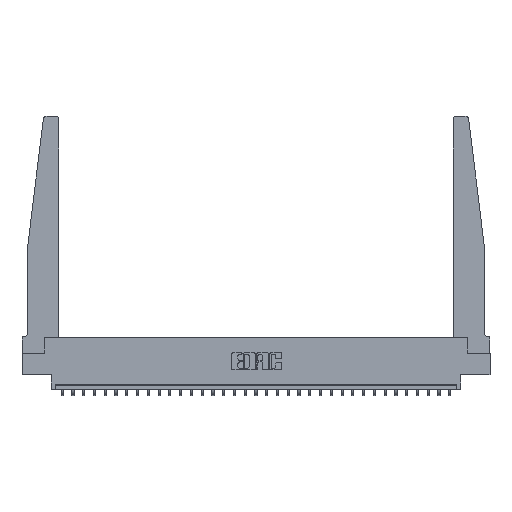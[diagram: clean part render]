
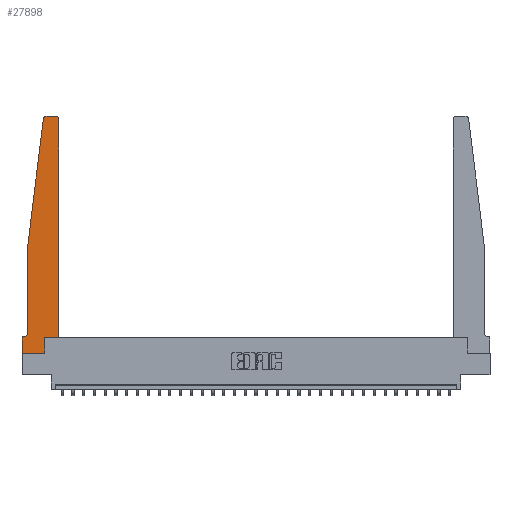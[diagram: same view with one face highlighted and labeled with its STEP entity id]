
A CAD part, top view. The second image highlights one B-rep face of the part: STEP entity #27898.
In plain terms, the highlighted planar face has unit normal (0, 0, 1).
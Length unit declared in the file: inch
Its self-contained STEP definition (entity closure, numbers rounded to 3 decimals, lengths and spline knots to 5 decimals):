
#23 = CARTESIAN_POINT ( 'NONE',  ( 0.425, 0.18, 0.37 ) ) ;
#372 = ORIENTED_EDGE ( 'NONE', *, *, #11865, .T. ) ;
#1064 = CARTESIAN_POINT ( 'NONE',  ( 0., 0., 0.37 ) ) ;
#1239 = CARTESIAN_POINT ( 'NONE',  ( 0.065, 0.1875, 0.37 ) ) ;
#1518 = VECTOR ( 'NONE', #21437, 39.37008 ) ;
#2028 = ORIENTED_EDGE ( 'NONE', *, *, #18009, .T. ) ;
#2218 = FACE_OUTER_BOUND ( 'NONE', #23320, .T. ) ;
#2490 = CARTESIAN_POINT ( 'NONE',  ( 0., 0., 0.37 ) ) ;
#2788 = CARTESIAN_POINT ( 'NONE',  ( 0.395, 2.72, 0.37 ) ) ;
#3418 = ORIENTED_EDGE ( 'NONE', *, *, #25724, .T. ) ;
#3942 = CIRCLE ( 'NONE', #22882, 0.03 ) ;
#4179 = CARTESIAN_POINT ( 'NONE',  ( 0.015, 0.2375, 0.37 ) ) ;
#5084 = DIRECTION ( 'NONE',  ( 1., 0., 0. ) ) ;
#5441 = CIRCLE ( 'NONE', #22124, 0.05 ) ;
#5722 = VERTEX_POINT ( 'NONE', #16955 ) ;
#6026 = VECTOR ( 'NONE', #18475, 39.37008 ) ;
#6123 = CARTESIAN_POINT ( 'NONE',  ( 0.425, 0.18, 0.37 ) ) ;
#6219 = CARTESIAN_POINT ( 'NONE',  ( 0.25, 2.75, 0.37 ) ) ;
#6423 = DIRECTION ( 'NONE',  ( -1., 0., 0. ) ) ;
#6855 = DIRECTION ( 'NONE',  ( 0., 0., 1. ) ) ;
#7719 = EDGE_CURVE ( 'NONE', #25180, #16531, #5441, .T. ) ;
#7782 = ORIENTED_EDGE ( 'NONE', *, *, #21812, .T. ) ;
#7826 = LINE ( 'NONE', #6219, #13737 ) ;
#7830 = VERTEX_POINT ( 'NONE', #23 ) ;
#8105 = EDGE_CURVE ( 'NONE', #7830, #5722, #19169, .T. ) ;
#8348 = CARTESIAN_POINT ( 'NONE',  ( 0.27653, 2.75, 0.37 ) ) ;
#8395 = DIRECTION ( 'NONE',  ( 0., 1., 0. ) ) ;
#9206 = EDGE_CURVE ( 'NONE', #5722, #25004, #3942, .T. ) ;
#9526 = VERTEX_POINT ( 'NONE', #17227 ) ;
#9772 = VERTEX_POINT ( 'NONE', #24638 ) ;
#10007 = DIRECTION ( 'NONE',  ( 0., -1., 0. ) ) ;
#10221 = ORIENTED_EDGE ( 'NONE', *, *, #28121, .T. ) ;
#10327 = AXIS2_PLACEMENT_3D ( 'NONE', #14369, #25313, #12283 ) ;
#10805 = CARTESIAN_POINT ( 'NONE',  ( 0.395, 2.75, 0.37 ) ) ;
#10913 = VERTEX_POINT ( 'NONE', #22232 ) ;
#11154 = ORIENTED_EDGE ( 'NONE', *, *, #18378, .T. ) ;
#11454 = CARTESIAN_POINT ( 'NONE',  ( 0.065, 0.2375, 0.37 ) ) ;
#11865 = EDGE_CURVE ( 'NONE', #23906, #16080, #24420, .T. ) ;
#12283 = DIRECTION ( 'NONE',  ( 1., 0., 0. ) ) ;
#12728 = VECTOR ( 'NONE', #16366, 39.37008 ) ;
#13045 = DIRECTION ( 'NONE',  ( 1., 0., 0. ) ) ;
#13374 = CARTESIAN_POINT ( 'NONE',  ( 0.2605, 0.18, 0.37 ) ) ;
#13397 = LINE ( 'NONE', #18623, #12728 ) ;
#13688 = ORIENTED_EDGE ( 'NONE', *, *, #9206, .T. ) ;
#13737 = VECTOR ( 'NONE', #17207, 39.37008 ) ;
#14150 = VECTOR ( 'NONE', #10007, 39.37008 ) ;
#14369 = CARTESIAN_POINT ( 'NONE',  ( 0., 0.1875, 0.37 ) ) ;
#14981 = AXIS2_PLACEMENT_3D ( 'NONE', #19977, #6855, #22171 ) ;
#16080 = VERTEX_POINT ( 'NONE', #18528 ) ;
#16322 = CARTESIAN_POINT ( 'NONE',  ( 0.065, 1.25, 0.37 ) ) ;
#16366 = DIRECTION ( 'NONE',  ( -0.122, -0.992, 0. ) ) ;
#16531 = VERTEX_POINT ( 'NONE', #20473 ) ;
#16798 = VERTEX_POINT ( 'NONE', #8348 ) ;
#16955 = CARTESIAN_POINT ( 'NONE',  ( 0.425, 2.72, 0.37 ) ) ;
#16969 = ORIENTED_EDGE ( 'NONE', *, *, #8105, .T. ) ;
#17141 = EDGE_CURVE ( 'NONE', #9526, #9772, #13397, .T. ) ;
#17207 = DIRECTION ( 'NONE',  ( -1., 0., 0. ) ) ;
#17227 = CARTESIAN_POINT ( 'NONE',  ( 0.24675, 2.72367, 0.37 ) ) ;
#17357 = EDGE_CURVE ( 'NONE', #25004, #16798, #7826, .T. ) ;
#17724 = LINE ( 'NONE', #16322, #6026 ) ;
#18009 = EDGE_CURVE ( 'NONE', #16798, #9526, #20432, .T. ) ;
#18269 = DIRECTION ( 'NONE',  ( 0., 0., 1. ) ) ;
#18298 = VECTOR ( 'NONE', #18857, 39.37008 ) ;
#18378 = EDGE_CURVE ( 'NONE', #22071, #7830, #27659, .T. ) ;
#18475 = DIRECTION ( 'NONE',  ( 0., -1., 0. ) ) ;
#18528 = CARTESIAN_POINT ( 'NONE',  ( 0.2605, 0., 0.37 ) ) ;
#18623 = CARTESIAN_POINT ( 'NONE',  ( 0.065, 1.25, 0.37 ) ) ;
#18857 = DIRECTION ( 'NONE',  ( -1., 0., 0. ) ) ;
#19037 = ORIENTED_EDGE ( 'NONE', *, *, #17357, .T. ) ;
#19125 = CARTESIAN_POINT ( 'NONE',  ( 0.425, 0.18, 0.37 ) ) ;
#19169 = LINE ( 'NONE', #6123, #1518 ) ;
#19564 = DIRECTION ( 'NONE',  ( 0., 0., -1. ) ) ;
#19977 = CARTESIAN_POINT ( 'NONE',  ( 0.27653, 2.72, 0.37 ) ) ;
#20013 = EDGE_CURVE ( 'NONE', #9772, #25180, #17724, .T. ) ;
#20081 = ORIENTED_EDGE ( 'NONE', *, *, #17141, .T. ) ;
#20432 = CIRCLE ( 'NONE', #14981, 0.03 ) ;
#20473 = CARTESIAN_POINT ( 'NONE',  ( 0.015, 0.1875, 0.37 ) ) ;
#20675 = PLANE ( 'NONE',  #10327 ) ;
#21437 = DIRECTION ( 'NONE',  ( 0., 1., 0. ) ) ;
#21776 = VECTOR ( 'NONE', #27968, 39.37008 ) ;
#21812 = EDGE_CURVE ( 'NONE', #16531, #10913, #23405, .T. ) ;
#22071 = VERTEX_POINT ( 'NONE', #13374 ) ;
#22124 = AXIS2_PLACEMENT_3D ( 'NONE', #4179, #19564, #6423 ) ;
#22171 = DIRECTION ( 'NONE',  ( 1., 0., 0. ) ) ;
#22232 = CARTESIAN_POINT ( 'NONE',  ( 0., 0.1875, 0.37 ) ) ;
#22882 = AXIS2_PLACEMENT_3D ( 'NONE', #2788, #18269, #5084 ) ;
#23320 = EDGE_LOOP ( 'NONE', ( #19037, #2028, #20081, #24105, #24560, #7782, #10221, #372, #3418, #11154, #16969, #13688 ) ) ;
#23405 = LINE ( 'NONE', #1239, #18298 ) ;
#23906 = VERTEX_POINT ( 'NONE', #2490 ) ;
#23951 = CARTESIAN_POINT ( 'NONE',  ( 0., 0., 0.37 ) ) ;
#24105 = ORIENTED_EDGE ( 'NONE', *, *, #20013, .T. ) ;
#24420 = LINE ( 'NONE', #23951, #25126 ) ;
#24560 = ORIENTED_EDGE ( 'NONE', *, *, #7719, .T. ) ;
#24638 = CARTESIAN_POINT ( 'NONE',  ( 0.065, 1.25, 0.37 ) ) ;
#25004 = VERTEX_POINT ( 'NONE', #10805 ) ;
#25046 = LINE ( 'NONE', #1064, #14150 ) ;
#25126 = VECTOR ( 'NONE', #13045, 39.37008 ) ;
#25180 = VERTEX_POINT ( 'NONE', #11454 ) ;
#25313 = DIRECTION ( 'NONE',  ( 0., 0., 1. ) ) ;
#25724 = EDGE_CURVE ( 'NONE', #16080, #22071, #28238, .T. ) ;
#25939 = CARTESIAN_POINT ( 'NONE',  ( 0.2605, 0.18, 0.37 ) ) ;
#27553 = VECTOR ( 'NONE', #8395, 39.37008 ) ;
#27659 = LINE ( 'NONE', #19125, #21776 ) ;
#27898 = ADVANCED_FACE ( 'NONE', ( #2218 ), #20675, .T. ) ;
#27968 = DIRECTION ( 'NONE',  ( 1., 0., 0. ) ) ;
#28121 = EDGE_CURVE ( 'NONE', #10913, #23906, #25046, .T. ) ;
#28238 = LINE ( 'NONE', #25939, #27553 ) ;
